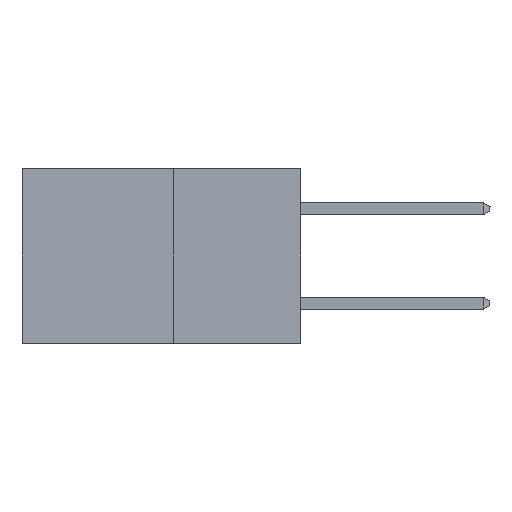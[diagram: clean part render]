
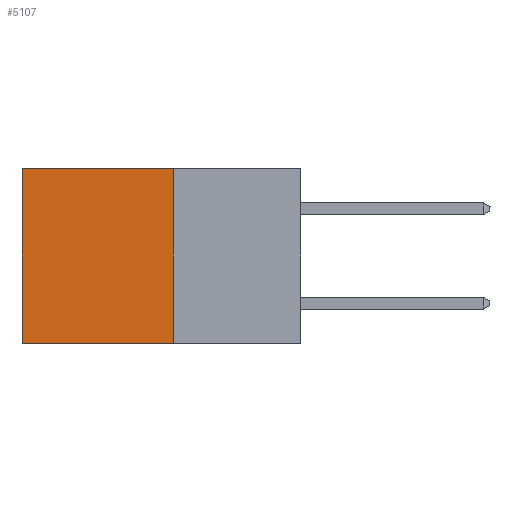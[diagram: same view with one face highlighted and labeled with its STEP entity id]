
A CAD part, left-side view. The second image highlights one B-rep face of the part: STEP entity #5107.
In plain terms, the highlighted planar face has unit normal (-1, 0, 0).
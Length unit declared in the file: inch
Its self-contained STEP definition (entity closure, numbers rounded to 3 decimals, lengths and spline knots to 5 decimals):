
#54 = EDGE_CURVE ( 'NONE', #3991, #1917, #2726, .T. ) ;
#120 = DIRECTION ( 'NONE',  ( 0., 1., 0. ) ) ;
#142 = VERTEX_POINT ( 'NONE', #5674 ) ;
#231 = EDGE_CURVE ( 'NONE', #3991, #4872, #1652, .T. ) ;
#303 = DIRECTION ( 'NONE',  ( 1., 0., 0. ) ) ;
#317 = PLANE ( 'NONE',  #1709 ) ;
#874 = VECTOR ( 'NONE', #1097, 39.37008 ) ;
#913 = DIRECTION ( 'NONE',  ( 0., 0., -1. ) ) ;
#1019 = CARTESIAN_POINT ( 'NONE',  ( 0.277, 0.27, -0.37 ) ) ;
#1048 = ORIENTED_EDGE ( 'NONE', *, *, #54, .T. ) ;
#1097 = DIRECTION ( 'NONE',  ( 0., 1., 0. ) ) ;
#1285 = CARTESIAN_POINT ( 'NONE',  ( 0.277, 0.27, -0.37 ) ) ;
#1652 = LINE ( 'NONE', #1019, #5071 ) ;
#1691 = EDGE_CURVE ( 'NONE', #1917, #142, #6265, .T. ) ;
#1709 = AXIS2_PLACEMENT_3D ( 'NONE', #1285, #303, #913 ) ;
#1917 = VERTEX_POINT ( 'NONE', #4410 ) ;
#2282 = EDGE_CURVE ( 'NONE', #4872, #142, #7631, .T. ) ;
#2582 = VECTOR ( 'NONE', #7313, 39.37008 ) ;
#2726 = LINE ( 'NONE', #3617, #874 ) ;
#3617 = CARTESIAN_POINT ( 'NONE',  ( 0.277, 0.27, 0. ) ) ;
#3945 = VECTOR ( 'NONE', #120, 39.37008 ) ;
#3991 = VERTEX_POINT ( 'NONE', #6632 ) ;
#4344 = ORIENTED_EDGE ( 'NONE', *, *, #231, .F. ) ;
#4410 = CARTESIAN_POINT ( 'NONE',  ( 0.277, 0.59, 0. ) ) ;
#4872 = VERTEX_POINT ( 'NONE', #7530 ) ;
#4922 = CARTESIAN_POINT ( 'NONE',  ( 0.277, 0.27, -0.37 ) ) ;
#5066 = FACE_OUTER_BOUND ( 'NONE', #8405, .T. ) ;
#5071 = VECTOR ( 'NONE', #6508, 39.37008 ) ;
#5107 = ADVANCED_FACE ( 'NONE', ( #5066 ), #317, .F. ) ;
#5615 = ORIENTED_EDGE ( 'NONE', *, *, #2282, .F. ) ;
#5674 = CARTESIAN_POINT ( 'NONE',  ( 0.277, 0.59, -0.37 ) ) ;
#6265 = LINE ( 'NONE', #8202, #2582 ) ;
#6508 = DIRECTION ( 'NONE',  ( 0., 0., -1. ) ) ;
#6632 = CARTESIAN_POINT ( 'NONE',  ( 0.277, 0.27, 0. ) ) ;
#7313 = DIRECTION ( 'NONE',  ( 0., 0., -1. ) ) ;
#7530 = CARTESIAN_POINT ( 'NONE',  ( 0.277, 0.27, -0.37 ) ) ;
#7631 = LINE ( 'NONE', #4922, #3945 ) ;
#8202 = CARTESIAN_POINT ( 'NONE',  ( 0.277, 0.59, -0.37 ) ) ;
#8282 = ORIENTED_EDGE ( 'NONE', *, *, #1691, .T. ) ;
#8405 = EDGE_LOOP ( 'NONE', ( #8282, #5615, #4344, #1048 ) ) ;
